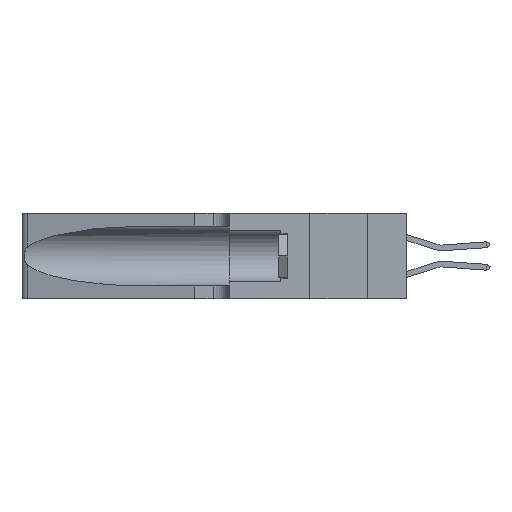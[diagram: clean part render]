
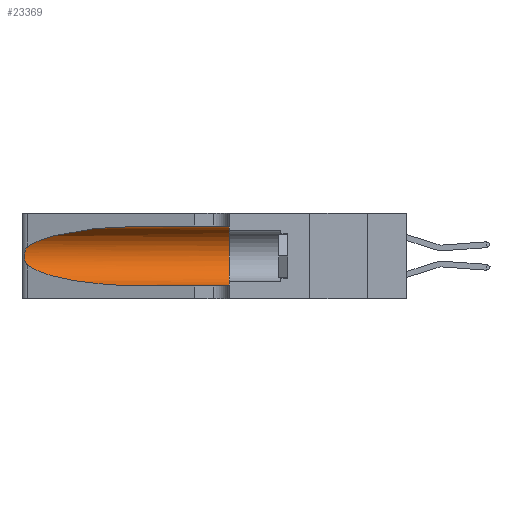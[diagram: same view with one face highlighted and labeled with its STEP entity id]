
A CAD part, left-side view. The second image highlights one B-rep face of the part: STEP entity #23369.
In plain terms, the highlighted cylindrical face has radius 3.308 mm (diameter 6.617 mm), a partial arc.
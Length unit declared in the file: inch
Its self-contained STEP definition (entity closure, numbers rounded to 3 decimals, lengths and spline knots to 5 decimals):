
#359 = B_SPLINE_CURVE_WITH_KNOTS ( 'NONE', 3,
 ( #25471, #28797, #8865, #32124, #12257, #35418, #15648, #38701, #19048, #42008, #22352, #2138, #25624, #5568 ),
 .UNSPECIFIED., .F., .F.,
 ( 4, 2, 2, 2, 2, 2, 4 ),
 ( 0., 0.00027, 0.00053, 0.00107, 0.0016, 0.00187, 0.00214 ),
 .UNSPECIFIED. ) ;
#1124 = ORIENTED_EDGE ( 'NONE', *, *, #18276, .T. ) ;
#2138 = CARTESIAN_POINT ( 'NONE',  ( 0.25639, 1.23186, 0.15144 ) ) ;
#3127 = CARTESIAN_POINT ( 'NONE',  ( 0.25487, 1.22718, 0.14631 ) ) ;
#3480 = CARTESIAN_POINT ( 'NONE',  ( 0.1305, 1.61858, 0.05475 ) ) ;
#4292 = VERTEX_POINT ( 'NONE', #9857 ) ;
#4461 = CARTESIAN_POINT ( 'NONE',  ( 0.1305, 1.61858, 0.31525 ) ) ;
#4892 = DIRECTION ( 'NONE',  ( 0., -1., 0. ) ) ;
#5045 = ORIENTED_EDGE ( 'NONE', *, *, #25590, .F. ) ;
#5568 = CARTESIAN_POINT ( 'NONE',  ( 0.25487, 1.22718, 0.14631 ) ) ;
#5933 = EDGE_CURVE ( 'NONE', #8847, #18597, #15788, .T. ) ;
#6566 = CARTESIAN_POINT ( 'NONE',  ( 0.2373, 1.15595, 0.08982 ) ) ;
#6785 = VECTOR ( 'NONE', #33548, 39.37008 ) ;
#7890 = ORIENTED_EDGE ( 'NONE', *, *, #5933, .T. ) ;
#8474 = CARTESIAN_POINT ( 'NONE',  ( 0.1305, 0.72297, 0.05475 ) ) ;
#8733 = EDGE_CURVE ( 'NONE', #32087, #4292, #30603, .T. ) ;
#8847 = VERTEX_POINT ( 'NONE', #8474 ) ;
#8865 = CARTESIAN_POINT ( 'NONE',  ( 0.25639, 1.23184, 0.21858 ) ) ;
#9857 = CARTESIAN_POINT ( 'NONE',  ( 0.1305, 0.35, 0.31525 ) ) ;
#10496 = CARTESIAN_POINT ( 'NONE',  ( 0.2373, 1.15595, 0.28018 ) ) ;
#11155 = VERTEX_POINT ( 'NONE', #20933 ) ;
#11435 = CARTESIAN_POINT ( 'NONE',  ( 0.1305, 0.35, 0.05475 ) ) ;
#12257 = CARTESIAN_POINT ( 'NONE',  ( 0.25854, 1.2359, 0.20912 ) ) ;
#15645 = ORIENTED_EDGE ( 'NONE', *, *, #30271, .T. ) ;
#15648 = CARTESIAN_POINT ( 'NONE',  ( 0.26075, 1.23896, 0.19203 ) ) ;
#15788 = LINE ( 'NONE', #3480, #6785 ) ;
#16764 = CARTESIAN_POINT ( 'NONE',  ( 0.18966, 0.96281, 0.05475 ) ) ;
#18146 = FACE_OUTER_BOUND ( 'NONE', #21865, .T. ) ;
#18276 = EDGE_CURVE ( 'NONE', #11155, #8847, #19412, .T. ) ;
#18527 = CARTESIAN_POINT ( 'NONE',  ( 0.1305, 0.35, 0.185 ) ) ;
#18597 = VERTEX_POINT ( 'NONE', #11435 ) ;
#19048 = CARTESIAN_POINT ( 'NONE',  ( 0.26017, 1.23833, 0.17102 ) ) ;
#19412 =( BOUNDED_CURVE ( )  B_SPLINE_CURVE ( 3, ( #3127, #6566, #16764, #39777 ),
 .UNSPECIFIED., .F., .F. ) 
 B_SPLINE_CURVE_WITH_KNOTS ( ( 4, 4 ),
 ( 3.44316, 4.71239 ),
 .UNSPECIFIED. ) 
 CURVE ( )  GEOMETRIC_REPRESENTATION_ITEM ( )  RATIONAL_B_SPLINE_CURVE ( ( 1., 0.87, 0.87, 1. ) ) 
 REPRESENTATION_ITEM ( '' )  );
#20486 = CARTESIAN_POINT ( 'NONE',  ( 0.1305, 0.72297, 0.31525 ) ) ;
#20933 = CARTESIAN_POINT ( 'NONE',  ( 0.25487, 1.22718, 0.14631 ) ) ;
#21018 = ORIENTED_EDGE ( 'NONE', *, *, #40311, .T. ) ;
#21686 = CARTESIAN_POINT ( 'NONE',  ( 0.1305, 1.61858, 0.185 ) ) ;
#21853 = DIRECTION ( 'NONE',  ( 0., 0., 1. ) ) ;
#21865 = EDGE_LOOP ( 'NONE', ( #15645, #21018, #1124, #7890, #5045, #25961 ) ) ;
#22352 = CARTESIAN_POINT ( 'NONE',  ( 0.25789, 1.23486, 0.15765 ) ) ;
#23151 = CARTESIAN_POINT ( 'NONE',  ( 0.25487, 1.22718, 0.22369 ) ) ;
#23369 = ADVANCED_FACE ( 'NONE', ( #18146 ), #24828, .F. ) ;
#24828 = CYLINDRICAL_SURFACE ( 'NONE', #37537, 0.13025 ) ;
#25471 = CARTESIAN_POINT ( 'NONE',  ( 0.25487, 1.22718, 0.22369 ) ) ;
#25590 = EDGE_CURVE ( 'NONE', #4292, #18597, #25669, .T. ) ;
#25624 = CARTESIAN_POINT ( 'NONE',  ( 0.25555, 1.22993, 0.14849 ) ) ;
#25669 = CIRCLE ( 'NONE', #35425, 0.13025 ) ;
#25888 = VERTEX_POINT ( 'NONE', #23151 ) ;
#25961 = ORIENTED_EDGE ( 'NONE', *, *, #8733, .F. ) ;
#28797 = CARTESIAN_POINT ( 'NONE',  ( 0.25555, 1.22994, 0.2215 ) ) ;
#30271 = EDGE_CURVE ( 'NONE', #32087, #25888, #31528, .T. ) ;
#30603 = LINE ( 'NONE', #4461, #37253 ) ;
#31320 = DIRECTION ( 'NONE',  ( 0., -1., 0. ) ) ;
#31528 =( BOUNDED_CURVE ( )  B_SPLINE_CURVE ( 3, ( #20486, #40146, #10496, #33712 ),
 .UNSPECIFIED., .F., .F. ) 
 B_SPLINE_CURVE_WITH_KNOTS ( ( 4, 4 ),
 ( 1.5708, 2.84003 ),
 .UNSPECIFIED. ) 
 CURVE ( )  GEOMETRIC_REPRESENTATION_ITEM ( )  RATIONAL_B_SPLINE_CURVE ( ( 1., 0.87, 0.87, 1. ) ) 
 REPRESENTATION_ITEM ( '' )  );
#32087 = VERTEX_POINT ( 'NONE', #33444 ) ;
#32124 = CARTESIAN_POINT ( 'NONE',  ( 0.25787, 1.23484, 0.2124 ) ) ;
#33444 = CARTESIAN_POINT ( 'NONE',  ( 0.1305, 0.72297, 0.31525 ) ) ;
#33548 = DIRECTION ( 'NONE',  ( 0., -1., 0. ) ) ;
#33712 = CARTESIAN_POINT ( 'NONE',  ( 0.25487, 1.22718, 0.22369 ) ) ;
#35418 = CARTESIAN_POINT ( 'NONE',  ( 0.26018, 1.23835, 0.19895 ) ) ;
#35425 = AXIS2_PLACEMENT_3D ( 'NONE', #18527, #41504, #21853 ) ;
#37253 = VECTOR ( 'NONE', #31320, 39.37008 ) ;
#37537 = AXIS2_PLACEMENT_3D ( 'NONE', #21686, #4892, #41338 ) ;
#38701 = CARTESIAN_POINT ( 'NONE',  ( 0.26075, 1.23896, 0.178 ) ) ;
#39777 = CARTESIAN_POINT ( 'NONE',  ( 0.1305, 0.72297, 0.05475 ) ) ;
#40146 = CARTESIAN_POINT ( 'NONE',  ( 0.18966, 0.96281, 0.31525 ) ) ;
#40311 = EDGE_CURVE ( 'NONE', #25888, #11155, #359, .T. ) ;
#41338 = DIRECTION ( 'NONE',  ( 0., 0., -1. ) ) ;
#41504 = DIRECTION ( 'NONE',  ( 0., 1., 0. ) ) ;
#42008 = CARTESIAN_POINT ( 'NONE',  ( 0.25856, 1.23593, 0.16098 ) ) ;
